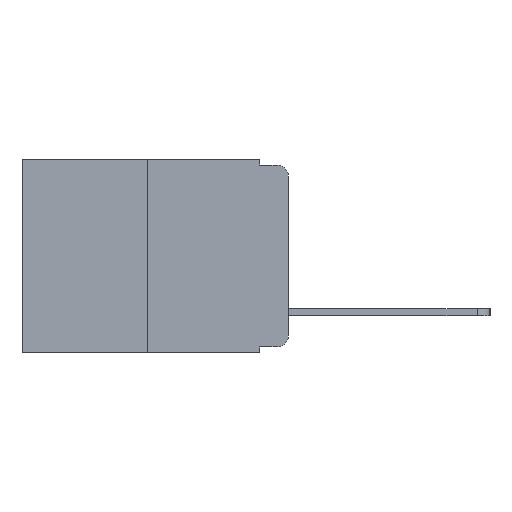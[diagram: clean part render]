
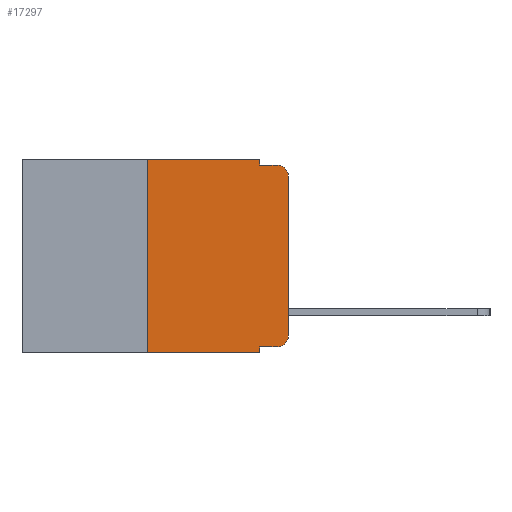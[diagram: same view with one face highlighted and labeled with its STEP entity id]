
A CAD part, left-side view. The second image highlights one B-rep face of the part: STEP entity #17297.
In plain terms, the highlighted planar face has unit normal (-1, 0, 0).
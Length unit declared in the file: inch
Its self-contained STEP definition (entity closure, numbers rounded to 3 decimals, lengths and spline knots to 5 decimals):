
#4 = ORIENTED_EDGE ( 'NONE', *, *, #10005, .T. ) ;
#1118 = CARTESIAN_POINT ( 'NONE',  ( 0., 0., 0. ) ) ;
#1226 = EDGE_CURVE ( 'NONE', #13663, #16942, #14224, .T. ) ;
#1271 = LINE ( 'NONE', #1915, #4630 ) ;
#1482 = LINE ( 'NONE', #15447, #5827 ) ;
#1485 = CARTESIAN_POINT ( 'NONE',  ( 0., 0.02, -0.333 ) ) ;
#1915 = CARTESIAN_POINT ( 'NONE',  ( 0., 0.25, 0. ) ) ;
#2612 = CIRCLE ( 'NONE', #10243, 0.02 ) ;
#2650 = VERTEX_POINT ( 'NONE', #14754 ) ;
#3009 = ORIENTED_EDGE ( 'NONE', *, *, #9712, .T. ) ;
#3161 = VERTEX_POINT ( 'NONE', #12507 ) ;
#3703 = CARTESIAN_POINT ( 'NONE',  ( 0., 0.051, 0. ) ) ;
#3719 = EDGE_CURVE ( 'NONE', #14731, #7607, #15771, .T. ) ;
#3815 = LINE ( 'NONE', #11818, #19544 ) ;
#3975 = DIRECTION ( 'NONE',  ( 0., 0., -1. ) ) ;
#4037 = EDGE_CURVE ( 'NONE', #14451, #3161, #14861, .T. ) ;
#4519 = DIRECTION ( 'NONE',  ( 0., -1., 0. ) ) ;
#4587 = CARTESIAN_POINT ( 'NONE',  ( 0., 0.051, -0.01 ) ) ;
#4630 = VECTOR ( 'NONE', #14354, 39.37008 ) ;
#4828 = CARTESIAN_POINT ( 'NONE',  ( 0., 0.02, -0.313 ) ) ;
#5165 = DIRECTION ( 'NONE',  ( 0., -1., 0. ) ) ;
#5376 = VECTOR ( 'NONE', #11797, 39.37008 ) ;
#5659 = EDGE_CURVE ( 'NONE', #17203, #13663, #3815, .T. ) ;
#5742 = ORIENTED_EDGE ( 'NONE', *, *, #19605, .F. ) ;
#5825 = CARTESIAN_POINT ( 'NONE',  ( 0., 0.051, -0.343 ) ) ;
#5827 = VECTOR ( 'NONE', #6324, 39.37008 ) ;
#5956 = DIRECTION ( 'NONE',  ( -1., 0., 0. ) ) ;
#6107 = VECTOR ( 'NONE', #4519, 39.37008 ) ;
#6324 = DIRECTION ( 'NONE',  ( 0., 0., -1. ) ) ;
#6405 = DIRECTION ( 'NONE',  ( 0., 0., -1. ) ) ;
#7187 = VERTEX_POINT ( 'NONE', #1485 ) ;
#7607 = VERTEX_POINT ( 'NONE', #5825 ) ;
#7926 = DIRECTION ( 'NONE',  ( 0., 0., 1. ) ) ;
#8204 = DIRECTION ( 'NONE',  ( 0., -1., 0. ) ) ;
#8355 = ORIENTED_EDGE ( 'NONE', *, *, #9531, .F. ) ;
#9303 = ORIENTED_EDGE ( 'NONE', *, *, #4037, .T. ) ;
#9531 = EDGE_CURVE ( 'NONE', #14731, #14787, #1271, .T. ) ;
#9707 = CARTESIAN_POINT ( 'NONE',  ( 0., 0.473, 0. ) ) ;
#9712 = EDGE_CURVE ( 'NONE', #2650, #7187, #13530, .T. ) ;
#10005 = EDGE_CURVE ( 'NONE', #7187, #14451, #20063, .T. ) ;
#10243 = AXIS2_PLACEMENT_3D ( 'NONE', #15079, #5956, #16591 ) ;
#10268 = CARTESIAN_POINT ( 'NONE',  ( 0., 0.051, -0.333 ) ) ;
#10504 = CARTESIAN_POINT ( 'NONE',  ( 0., 0.25, 0. ) ) ;
#10512 = CARTESIAN_POINT ( 'NONE',  ( 0., 0.02, -0.01 ) ) ;
#10525 = ORIENTED_EDGE ( 'NONE', *, *, #1226, .F. ) ;
#11017 = ORIENTED_EDGE ( 'NONE', *, *, #14471, .F. ) ;
#11332 = VECTOR ( 'NONE', #7926, 39.37008 ) ;
#11692 = PLANE ( 'NONE',  #17732 ) ;
#11786 = VECTOR ( 'NONE', #5165, 39.37008 ) ;
#11797 = DIRECTION ( 'NONE',  ( 0., -1., 0. ) ) ;
#11818 = CARTESIAN_POINT ( 'NONE',  ( 0., 0.051, 0. ) ) ;
#11901 = CARTESIAN_POINT ( 'NONE',  ( 0., 0.25, -0.343 ) ) ;
#12395 = CARTESIAN_POINT ( 'NONE',  ( 0., 0.473, -0.343 ) ) ;
#12507 = CARTESIAN_POINT ( 'NONE',  ( 0., 0., -0.03 ) ) ;
#12528 = FACE_OUTER_BOUND ( 'NONE', #16909, .T. ) ;
#12562 = EDGE_CURVE ( 'NONE', #3161, #16942, #2612, .T. ) ;
#12684 = ORIENTED_EDGE ( 'NONE', *, *, #3719, .T. ) ;
#13221 = DIRECTION ( 'NONE',  ( 1., 0., 0. ) ) ;
#13332 = DIRECTION ( 'NONE',  ( 0., 0., -1. ) ) ;
#13530 = LINE ( 'NONE', #10268, #5376 ) ;
#13663 = VERTEX_POINT ( 'NONE', #16161 ) ;
#14224 = LINE ( 'NONE', #4587, #6107 ) ;
#14301 = ORIENTED_EDGE ( 'NONE', *, *, #5659, .F. ) ;
#14354 = DIRECTION ( 'NONE',  ( 0., 0., 1. ) ) ;
#14451 = VERTEX_POINT ( 'NONE', #17228 ) ;
#14471 = EDGE_CURVE ( 'NONE', #14787, #17203, #14767, .T. ) ;
#14626 = AXIS2_PLACEMENT_3D ( 'NONE', #4828, #15526, #6405 ) ;
#14731 = VERTEX_POINT ( 'NONE', #11901 ) ;
#14754 = CARTESIAN_POINT ( 'NONE',  ( 0., 0.051, -0.333 ) ) ;
#14767 = LINE ( 'NONE', #9707, #17340 ) ;
#14787 = VERTEX_POINT ( 'NONE', #10504 ) ;
#14861 = LINE ( 'NONE', #1118, #11332 ) ;
#15079 = CARTESIAN_POINT ( 'NONE',  ( 0., 0.02, -0.03 ) ) ;
#15447 = CARTESIAN_POINT ( 'NONE',  ( 0., 0.051, 0. ) ) ;
#15526 = DIRECTION ( 'NONE',  ( -1., 0., 0. ) ) ;
#15771 = LINE ( 'NONE', #12395, #11786 ) ;
#16092 = CARTESIAN_POINT ( 'NONE',  ( 0., 0.473, 0. ) ) ;
#16161 = CARTESIAN_POINT ( 'NONE',  ( 0., 0.051, -0.01 ) ) ;
#16173 = ORIENTED_EDGE ( 'NONE', *, *, #12562, .T. ) ;
#16591 = DIRECTION ( 'NONE',  ( 0., 0., -1. ) ) ;
#16909 = EDGE_LOOP ( 'NONE', ( #9303, #16173, #10525, #14301, #11017, #8355, #12684, #5742, #3009, #4 ) ) ;
#16942 = VERTEX_POINT ( 'NONE', #10512 ) ;
#17203 = VERTEX_POINT ( 'NONE', #3703 ) ;
#17228 = CARTESIAN_POINT ( 'NONE',  ( 0., 0., -0.313 ) ) ;
#17297 = ADVANCED_FACE ( 'NONE', ( #12528 ), #11692, .F. ) ;
#17340 = VECTOR ( 'NONE', #8204, 39.37008 ) ;
#17732 = AXIS2_PLACEMENT_3D ( 'NONE', #16092, #13221, #3975 ) ;
#19544 = VECTOR ( 'NONE', #13332, 39.37008 ) ;
#19605 = EDGE_CURVE ( 'NONE', #2650, #7607, #1482, .T. ) ;
#20063 = CIRCLE ( 'NONE', #14626, 0.02 ) ;
